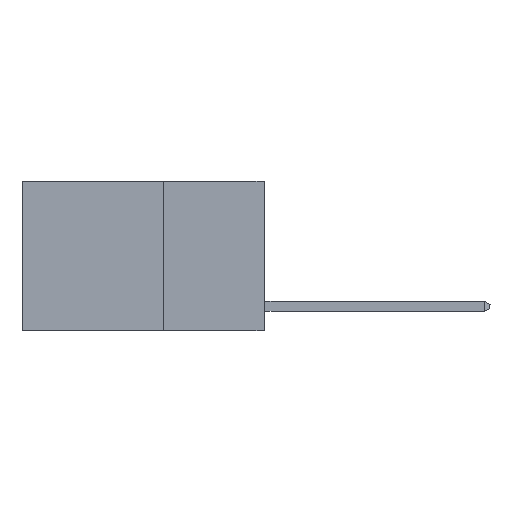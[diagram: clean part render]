
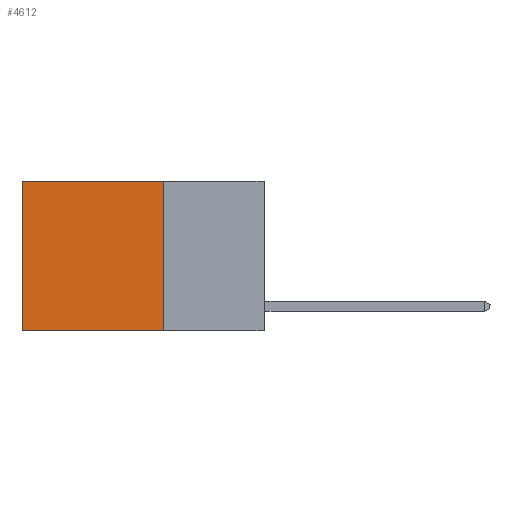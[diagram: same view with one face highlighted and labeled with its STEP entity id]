
A CAD part, left-side view. The second image highlights one B-rep face of the part: STEP entity #4612.
In plain terms, the highlighted planar face has unit normal (-1, 0, 0).
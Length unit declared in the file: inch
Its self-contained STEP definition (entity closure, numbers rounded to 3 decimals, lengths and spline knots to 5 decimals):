
#452 = CARTESIAN_POINT ( 'NONE',  ( 0.2625, 0.6, 0. ) ) ;
#825 = DIRECTION ( 'NONE',  ( 0., 1., 0. ) ) ;
#1106 = VECTOR ( 'NONE', #11679, 39.37008 ) ;
#1544 = ORIENTED_EDGE ( 'NONE', *, *, #7620, .T. ) ;
#2253 = DIRECTION ( 'NONE',  ( 0., 0., -1. ) ) ;
#3131 = VERTEX_POINT ( 'NONE', #9329 ) ;
#4238 = CARTESIAN_POINT ( 'NONE',  ( 0.2625, 0.25, -0.37 ) ) ;
#4276 = ORIENTED_EDGE ( 'NONE', *, *, #21368, .T. ) ;
#4347 = ORIENTED_EDGE ( 'NONE', *, *, #19858, .F. ) ;
#4612 = ADVANCED_FACE ( 'NONE', ( #9829 ), #6507, .F. ) ;
#4903 = LINE ( 'NONE', #13937, #13743 ) ;
#5744 = VECTOR ( 'NONE', #825, 39.37008 ) ;
#6507 = PLANE ( 'NONE',  #10529 ) ;
#7346 = CARTESIAN_POINT ( 'NONE',  ( 0.2625, 0.6, -0.37 ) ) ;
#7445 = LINE ( 'NONE', #10592, #15673 ) ;
#7620 = EDGE_CURVE ( 'NONE', #20922, #19679, #7445, .T. ) ;
#7654 = VERTEX_POINT ( 'NONE', #17228 ) ;
#9329 = CARTESIAN_POINT ( 'NONE',  ( 0.2625, 0.25, -0.37 ) ) ;
#9829 = FACE_OUTER_BOUND ( 'NONE', #15712, .T. ) ;
#9851 = DIRECTION ( 'NONE',  ( 0., 0., -1. ) ) ;
#10529 = AXIS2_PLACEMENT_3D ( 'NONE', #17998, #19626, #9851 ) ;
#10592 = CARTESIAN_POINT ( 'NONE',  ( 0.2625, 0.6, 0. ) ) ;
#11679 = DIRECTION ( 'NONE',  ( 0., 1., 0. ) ) ;
#12420 = ORIENTED_EDGE ( 'NONE', *, *, #19155, .F. ) ;
#13743 = VECTOR ( 'NONE', #2253, 39.37008 ) ;
#13937 = CARTESIAN_POINT ( 'NONE',  ( 0.2625, 0.25, 0. ) ) ;
#14449 = LINE ( 'NONE', #21423, #1106 ) ;
#15058 = LINE ( 'NONE', #4238, #5744 ) ;
#15673 = VECTOR ( 'NONE', #17160, 39.37008 ) ;
#15712 = EDGE_LOOP ( 'NONE', ( #1544, #12420, #4347, #4276 ) ) ;
#17160 = DIRECTION ( 'NONE',  ( 0., 0., -1. ) ) ;
#17228 = CARTESIAN_POINT ( 'NONE',  ( 0.2625, 0.25, 0. ) ) ;
#17998 = CARTESIAN_POINT ( 'NONE',  ( 0.2625, 0.25, 0. ) ) ;
#19155 = EDGE_CURVE ( 'NONE', #3131, #19679, #15058, .T. ) ;
#19626 = DIRECTION ( 'NONE',  ( 1., 0., 0. ) ) ;
#19679 = VERTEX_POINT ( 'NONE', #7346 ) ;
#19858 = EDGE_CURVE ( 'NONE', #7654, #3131, #4903, .T. ) ;
#20922 = VERTEX_POINT ( 'NONE', #452 ) ;
#21368 = EDGE_CURVE ( 'NONE', #7654, #20922, #14449, .T. ) ;
#21423 = CARTESIAN_POINT ( 'NONE',  ( 0.2625, 0.25, 0. ) ) ;
